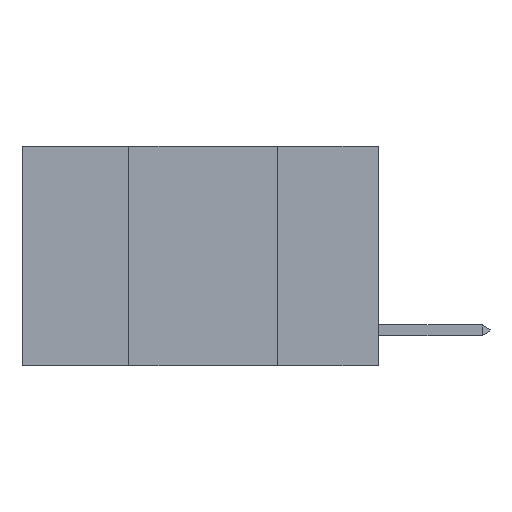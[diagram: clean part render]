
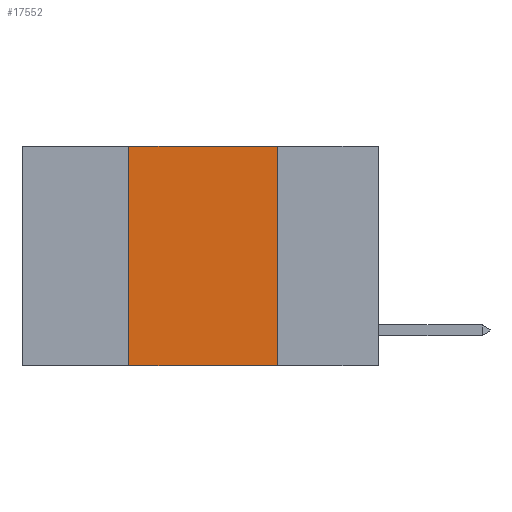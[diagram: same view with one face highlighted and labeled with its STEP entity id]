
A CAD part, left-side view. The second image highlights one B-rep face of the part: STEP entity #17552.
In plain terms, the highlighted planar face has unit normal (-1, 0, 0).
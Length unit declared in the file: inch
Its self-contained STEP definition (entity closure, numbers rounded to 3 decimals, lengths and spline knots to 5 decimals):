
#163 = LINE ( 'NONE', #4567, #19613 ) ;
#1741 = EDGE_CURVE ( 'NONE', #4900, #18249, #163, .T. ) ;
#1815 = CARTESIAN_POINT ( 'NONE',  ( 0., 0.6, 0. ) ) ;
#2134 = VECTOR ( 'NONE', #5655, 39.37008 ) ;
#2758 = DIRECTION ( 'NONE',  ( 0., 0., -1. ) ) ;
#3048 = CARTESIAN_POINT ( 'NONE',  ( 0., 0.42, 0. ) ) ;
#3128 = DIRECTION ( 'NONE',  ( 0., -1., 0. ) ) ;
#3258 = AXIS2_PLACEMENT_3D ( 'NONE', #1815, #14601, #3647 ) ;
#3647 = DIRECTION ( 'NONE',  ( 0., 0., -1. ) ) ;
#4090 = CARTESIAN_POINT ( 'NONE',  ( 0., 0.17, -0.37 ) ) ;
#4567 = CARTESIAN_POINT ( 'NONE',  ( 0., 0.17, 0. ) ) ;
#4900 = VERTEX_POINT ( 'NONE', #7475 ) ;
#5655 = DIRECTION ( 'NONE',  ( 0., -1., 0. ) ) ;
#6221 = EDGE_CURVE ( 'NONE', #14867, #18249, #6970, .T. ) ;
#6970 = LINE ( 'NONE', #18465, #2134 ) ;
#7475 = CARTESIAN_POINT ( 'NONE',  ( 0., 0.17, 0. ) ) ;
#9148 = CARTESIAN_POINT ( 'NONE',  ( 0., 0.42, 0. ) ) ;
#10523 = EDGE_LOOP ( 'NONE', ( #19147, #20763, #22333, #10829 ) ) ;
#10829 = ORIENTED_EDGE ( 'NONE', *, *, #6221, .T. ) ;
#13498 = VERTEX_POINT ( 'NONE', #3048 ) ;
#14601 = DIRECTION ( 'NONE',  ( 1., 0., 0. ) ) ;
#14867 = VERTEX_POINT ( 'NONE', #18422 ) ;
#15058 = FACE_OUTER_BOUND ( 'NONE', #10523, .T. ) ;
#16510 = DIRECTION ( 'NONE',  ( 0., 0., 1. ) ) ;
#17552 = ADVANCED_FACE ( 'NONE', ( #15058 ), #20023, .F. ) ;
#17588 = VECTOR ( 'NONE', #3128, 39.37008 ) ;
#17608 = LINE ( 'NONE', #9148, #21859 ) ;
#18117 = EDGE_CURVE ( 'NONE', #14867, #13498, #17608, .T. ) ;
#18146 = LINE ( 'NONE', #23149, #17588 ) ;
#18249 = VERTEX_POINT ( 'NONE', #4090 ) ;
#18422 = CARTESIAN_POINT ( 'NONE',  ( 0., 0.42, -0.37 ) ) ;
#18465 = CARTESIAN_POINT ( 'NONE',  ( 0., 0.6, -0.37 ) ) ;
#18549 = EDGE_CURVE ( 'NONE', #13498, #4900, #18146, .T. ) ;
#19147 = ORIENTED_EDGE ( 'NONE', *, *, #1741, .F. ) ;
#19613 = VECTOR ( 'NONE', #2758, 39.37008 ) ;
#20023 = PLANE ( 'NONE',  #3258 ) ;
#20763 = ORIENTED_EDGE ( 'NONE', *, *, #18549, .F. ) ;
#21859 = VECTOR ( 'NONE', #16510, 39.37008 ) ;
#22333 = ORIENTED_EDGE ( 'NONE', *, *, #18117, .F. ) ;
#23149 = CARTESIAN_POINT ( 'NONE',  ( 0., 0.6, 0. ) ) ;
